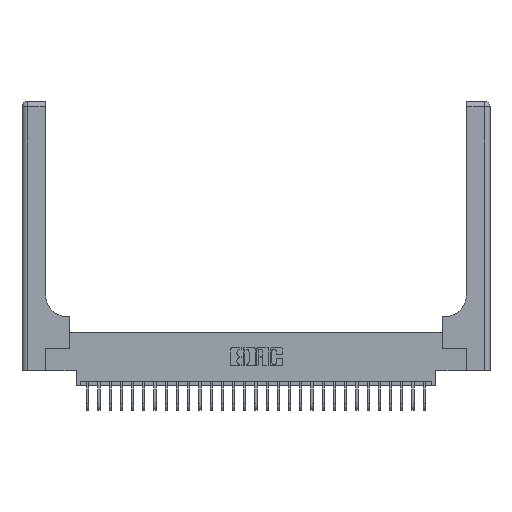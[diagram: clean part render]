
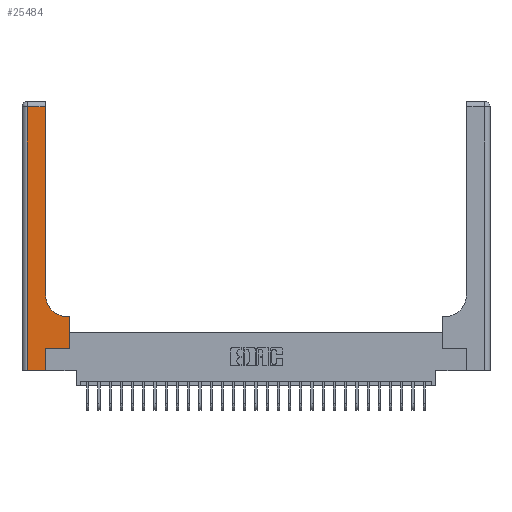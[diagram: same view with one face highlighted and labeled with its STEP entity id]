
A CAD part, top view. The second image highlights one B-rep face of the part: STEP entity #25484.
In plain terms, the highlighted planar face has unit normal (0, 0, 1).
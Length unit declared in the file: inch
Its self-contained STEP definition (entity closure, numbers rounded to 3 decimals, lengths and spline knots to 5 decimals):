
#184 = DIRECTION ( 'NONE',  ( 0., -1., 0. ) ) ;
#390 = LINE ( 'NONE', #17356, #10654 ) ;
#696 = FACE_OUTER_BOUND ( 'NONE', #3678, .T. ) ;
#841 = CARTESIAN_POINT ( 'NONE',  ( 0.51, 0.85, 0.37 ) ) ;
#944 = VECTOR ( 'NONE', #1496, 39.37008 ) ;
#1496 = DIRECTION ( 'NONE',  ( -1., 0., 0. ) ) ;
#2596 = CARTESIAN_POINT ( 'NONE',  ( 0., 0., 0.37 ) ) ;
#2882 = DIRECTION ( 'NONE',  ( 1., 0., 0. ) ) ;
#2917 = CARTESIAN_POINT ( 'NONE',  ( 0.26, 2.94, 0.37 ) ) ;
#3085 = VECTOR ( 'NONE', #184, 39.37008 ) ;
#3122 = VERTEX_POINT ( 'NONE', #3169 ) ;
#3169 = CARTESIAN_POINT ( 'NONE',  ( 0.528, 0.25, 0.37 ) ) ;
#3345 = CARTESIAN_POINT ( 'NONE',  ( 0.265, 0.25, 0.37 ) ) ;
#3559 = EDGE_CURVE ( 'NONE', #5041, #23712, #14493, .T. ) ;
#3678 = EDGE_LOOP ( 'NONE', ( #6215, #22223, #6857, #18185, #8151, #8777, #14128, #3938, #20659 ) ) ;
#3938 = ORIENTED_EDGE ( 'NONE', *, *, #20916, .T. ) ;
#4404 = CARTESIAN_POINT ( 'NONE',  ( 0.51, 0.6, 0.37 ) ) ;
#4481 = CARTESIAN_POINT ( 'NONE',  ( 0.06, 0., 0.37 ) ) ;
#4879 = DIRECTION ( 'NONE',  ( -1., 0., 0. ) ) ;
#5011 = PLANE ( 'NONE',  #14441 ) ;
#5041 = VERTEX_POINT ( 'NONE', #4404 ) ;
#5139 = EDGE_CURVE ( 'NONE', #15968, #23612, #8181, .T. ) ;
#5924 = EDGE_CURVE ( 'NONE', #23612, #25259, #390, .T. ) ;
#5980 = VERTEX_POINT ( 'NONE', #9502 ) ;
#6215 = ORIENTED_EDGE ( 'NONE', *, *, #11995, .T. ) ;
#6612 = LINE ( 'NONE', #9839, #11359 ) ;
#6857 = ORIENTED_EDGE ( 'NONE', *, *, #15909, .T. ) ;
#7128 = VECTOR ( 'NONE', #17526, 39.37008 ) ;
#7656 = DIRECTION ( 'NONE',  ( 0., 1., 0. ) ) ;
#8151 = ORIENTED_EDGE ( 'NONE', *, *, #5924, .T. ) ;
#8181 = LINE ( 'NONE', #2596, #22867 ) ;
#8327 = AXIS2_PLACEMENT_3D ( 'NONE', #841, #15061, #2882 ) ;
#8667 = VECTOR ( 'NONE', #7656, 39.37008 ) ;
#8777 = ORIENTED_EDGE ( 'NONE', *, *, #10969, .T. ) ;
#9172 = CARTESIAN_POINT ( 'NONE',  ( 0., 3., 0.37 ) ) ;
#9237 = LINE ( 'NONE', #22452, #3085 ) ;
#9414 = DIRECTION ( 'NONE',  ( 0., 1., 0. ) ) ;
#9502 = CARTESIAN_POINT ( 'NONE',  ( 0.06, 2.94, 0.37 ) ) ;
#9839 = CARTESIAN_POINT ( 'NONE',  ( 0.528, 0.25, 0.37 ) ) ;
#10401 = CARTESIAN_POINT ( 'NONE',  ( 0.265, 0.25, 0.37 ) ) ;
#10654 = VECTOR ( 'NONE', #9414, 39.37008 ) ;
#10844 = DIRECTION ( 'NONE',  ( 1., 0., 0. ) ) ;
#10969 = EDGE_CURVE ( 'NONE', #25259, #3122, #21236, .T. ) ;
#11169 = DIRECTION ( 'NONE',  ( -1., 0., 0. ) ) ;
#11359 = VECTOR ( 'NONE', #11848, 39.37008 ) ;
#11820 = LINE ( 'NONE', #14983, #23049 ) ;
#11848 = DIRECTION ( 'NONE',  ( 0., 1., 0. ) ) ;
#11995 = EDGE_CURVE ( 'NONE', #23712, #14345, #19308, .T. ) ;
#13713 = CARTESIAN_POINT ( 'NONE',  ( 0., 2.94, 0.37 ) ) ;
#14128 = ORIENTED_EDGE ( 'NONE', *, *, #16901, .T. ) ;
#14345 = VERTEX_POINT ( 'NONE', #2917 ) ;
#14441 = AXIS2_PLACEMENT_3D ( 'NONE', #9172, #23120, #11169 ) ;
#14493 = CIRCLE ( 'NONE', #8327, 0.25 ) ;
#14508 = EDGE_CURVE ( 'NONE', #14345, #5980, #16498, .T. ) ;
#14983 = CARTESIAN_POINT ( 'NONE',  ( 0.26, 0.6, 0.37 ) ) ;
#15061 = DIRECTION ( 'NONE',  ( 0., 0., -1. ) ) ;
#15808 = CARTESIAN_POINT ( 'NONE',  ( 0.265, 0., 0.37 ) ) ;
#15909 = EDGE_CURVE ( 'NONE', #5980, #15968, #9237, .T. ) ;
#15925 = VERTEX_POINT ( 'NONE', #16512 ) ;
#15968 = VERTEX_POINT ( 'NONE', #4481 ) ;
#16498 = LINE ( 'NONE', #13713, #944 ) ;
#16512 = CARTESIAN_POINT ( 'NONE',  ( 0.528, 0.6, 0.37 ) ) ;
#16901 = EDGE_CURVE ( 'NONE', #3122, #15925, #6612, .T. ) ;
#17356 = CARTESIAN_POINT ( 'NONE',  ( 0.265, 0., 0.37 ) ) ;
#17526 = DIRECTION ( 'NONE',  ( 1., 0., 0. ) ) ;
#18185 = ORIENTED_EDGE ( 'NONE', *, *, #5139, .T. ) ;
#19308 = LINE ( 'NONE', #21664, #8667 ) ;
#20659 = ORIENTED_EDGE ( 'NONE', *, *, #3559, .T. ) ;
#20916 = EDGE_CURVE ( 'NONE', #15925, #5041, #11820, .T. ) ;
#21236 = LINE ( 'NONE', #3345, #7128 ) ;
#21664 = CARTESIAN_POINT ( 'NONE',  ( 0.26, 3., 0.37 ) ) ;
#22223 = ORIENTED_EDGE ( 'NONE', *, *, #14508, .T. ) ;
#22452 = CARTESIAN_POINT ( 'NONE',  ( 0.06, 3., 0.37 ) ) ;
#22867 = VECTOR ( 'NONE', #10844, 39.37008 ) ;
#23049 = VECTOR ( 'NONE', #4879, 39.37008 ) ;
#23120 = DIRECTION ( 'NONE',  ( 0., 0., -1. ) ) ;
#23395 = CARTESIAN_POINT ( 'NONE',  ( 0.26, 0.85, 0.37 ) ) ;
#23612 = VERTEX_POINT ( 'NONE', #15808 ) ;
#23712 = VERTEX_POINT ( 'NONE', #23395 ) ;
#25259 = VERTEX_POINT ( 'NONE', #10401 ) ;
#25484 = ADVANCED_FACE ( 'NONE', ( #696 ), #5011, .F. ) ;
